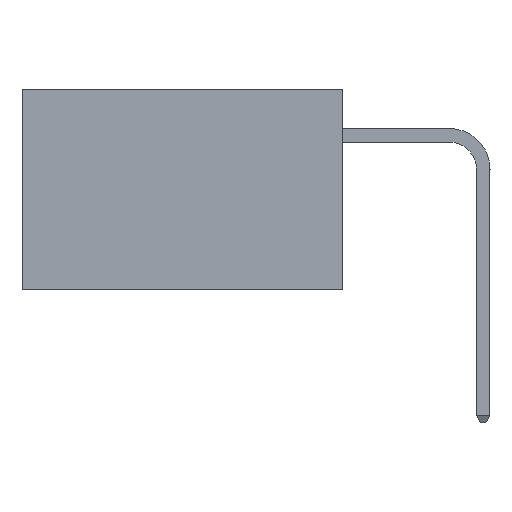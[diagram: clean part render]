
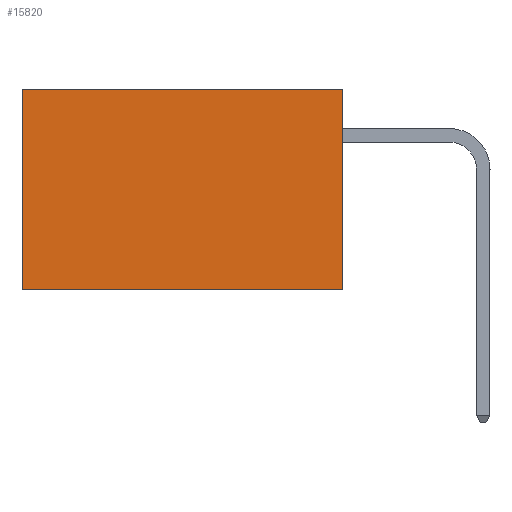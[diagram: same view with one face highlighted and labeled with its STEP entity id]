
A CAD part, left-side view. The second image highlights one B-rep face of the part: STEP entity #15820.
In plain terms, the highlighted planar face has unit normal (-1, 0, 0).
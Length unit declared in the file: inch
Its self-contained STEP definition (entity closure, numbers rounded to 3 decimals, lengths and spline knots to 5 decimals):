
#660 = VECTOR ( 'NONE', #5322, 39.37008 ) ;
#953 = EDGE_CURVE ( 'NONE', #7788, #7279, #16198, .T. ) ;
#998 = CARTESIAN_POINT ( 'NONE',  ( 0.277, 0., 0. ) ) ;
#2460 = CARTESIAN_POINT ( 'NONE',  ( 0.277, 0.59, -0.37 ) ) ;
#3153 = DIRECTION ( 'NONE',  ( 0., 0., -1. ) ) ;
#3157 = PLANE ( 'NONE',  #6641 ) ;
#4440 = CARTESIAN_POINT ( 'NONE',  ( 0.277, 0., -0.37 ) ) ;
#4630 = ORIENTED_EDGE ( 'NONE', *, *, #14873, .F. ) ;
#4842 = VERTEX_POINT ( 'NONE', #6569 ) ;
#5322 = DIRECTION ( 'NONE',  ( 0., 1., 0. ) ) ;
#6346 = FACE_OUTER_BOUND ( 'NONE', #6573, .T. ) ;
#6569 = CARTESIAN_POINT ( 'NONE',  ( 0.277, 0., -0.37 ) ) ;
#6573 = EDGE_LOOP ( 'NONE', ( #15344, #4630, #13669, #12068 ) ) ;
#6641 = AXIS2_PLACEMENT_3D ( 'NONE', #4440, #15517, #8238 ) ;
#7279 = VERTEX_POINT ( 'NONE', #13322 ) ;
#7788 = VERTEX_POINT ( 'NONE', #9276 ) ;
#8238 = DIRECTION ( 'NONE',  ( 0., 0., -1. ) ) ;
#8519 = CARTESIAN_POINT ( 'NONE',  ( 0.277, 0., -0.37 ) ) ;
#9276 = CARTESIAN_POINT ( 'NONE',  ( 0.277, 0., 0. ) ) ;
#9793 = LINE ( 'NONE', #8519, #13046 ) ;
#10719 = CARTESIAN_POINT ( 'NONE',  ( 0.277, 0.59, -0.37 ) ) ;
#11067 = DIRECTION ( 'NONE',  ( 0., 0., -1. ) ) ;
#12068 = ORIENTED_EDGE ( 'NONE', *, *, #953, .T. ) ;
#12289 = VECTOR ( 'NONE', #3153, 39.37008 ) ;
#12534 = EDGE_CURVE ( 'NONE', #7788, #4842, #9793, .T. ) ;
#12739 = VECTOR ( 'NONE', #15523, 39.37008 ) ;
#13044 = EDGE_CURVE ( 'NONE', #7279, #13368, #15777, .T. ) ;
#13046 = VECTOR ( 'NONE', #11067, 39.37008 ) ;
#13322 = CARTESIAN_POINT ( 'NONE',  ( 0.277, 0.59, 0. ) ) ;
#13368 = VERTEX_POINT ( 'NONE', #2460 ) ;
#13669 = ORIENTED_EDGE ( 'NONE', *, *, #12534, .F. ) ;
#14075 = LINE ( 'NONE', #15048, #660 ) ;
#14873 = EDGE_CURVE ( 'NONE', #4842, #13368, #14075, .T. ) ;
#15048 = CARTESIAN_POINT ( 'NONE',  ( 0.277, 0., -0.37 ) ) ;
#15344 = ORIENTED_EDGE ( 'NONE', *, *, #13044, .T. ) ;
#15517 = DIRECTION ( 'NONE',  ( 1., 0., 0. ) ) ;
#15523 = DIRECTION ( 'NONE',  ( 0., 1., 0. ) ) ;
#15777 = LINE ( 'NONE', #10719, #12289 ) ;
#15820 = ADVANCED_FACE ( 'NONE', ( #6346 ), #3157, .F. ) ;
#16198 = LINE ( 'NONE', #998, #12739 ) ;
